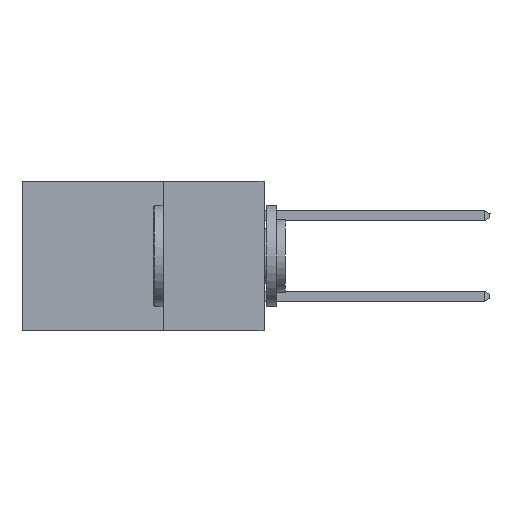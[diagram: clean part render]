
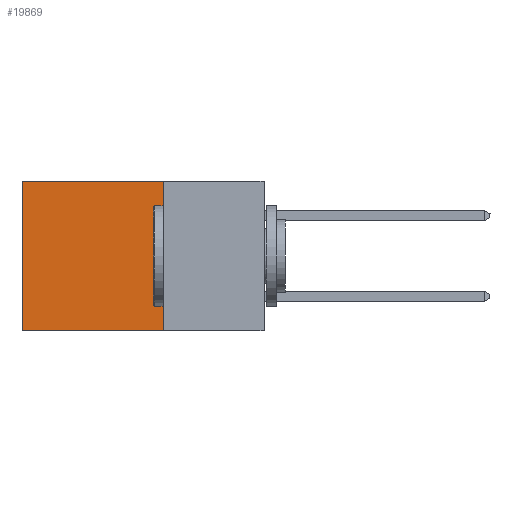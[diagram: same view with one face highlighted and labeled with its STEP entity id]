
A CAD part, left-side view. The second image highlights one B-rep face of the part: STEP entity #19869.
In plain terms, the highlighted planar face has unit normal (-1, 0, 0).
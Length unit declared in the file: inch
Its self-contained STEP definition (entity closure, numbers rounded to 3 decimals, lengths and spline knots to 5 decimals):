
#702 = CARTESIAN_POINT ( 'NONE',  ( 0.298, 0.25, 0. ) ) ;
#1252 = CARTESIAN_POINT ( 'NONE',  ( 0.298, 0.25, 0. ) ) ;
#1754 = ORIENTED_EDGE ( 'NONE', *, *, #15836, .T. ) ;
#6641 = EDGE_LOOP ( 'NONE', ( #19801, #10557, #20972, #1754 ) ) ;
#7192 = DIRECTION ( 'NONE',  ( 0., 0., -1. ) ) ;
#8201 = LINE ( 'NONE', #23012, #13774 ) ;
#8579 = LINE ( 'NONE', #20771, #9980 ) ;
#9673 = LINE ( 'NONE', #11593, #13516 ) ;
#9980 = VECTOR ( 'NONE', #27638, 39.37008 ) ;
#10557 = ORIENTED_EDGE ( 'NONE', *, *, #11553, .F. ) ;
#10643 = FACE_OUTER_BOUND ( 'NONE', #6641, .T. ) ;
#11553 = EDGE_CURVE ( 'NONE', #19592, #14748, #8579, .T. ) ;
#11593 = CARTESIAN_POINT ( 'NONE',  ( 0.298, 0.25, 0. ) ) ;
#12552 = CARTESIAN_POINT ( 'NONE',  ( 0.298, 0.25, -0.37 ) ) ;
#13516 = VECTOR ( 'NONE', #7192, 39.37008 ) ;
#13774 = VECTOR ( 'NONE', #25416, 39.37008 ) ;
#14577 = DIRECTION ( 'NONE',  ( 1., 0., 0. ) ) ;
#14748 = VERTEX_POINT ( 'NONE', #20721 ) ;
#14956 = LINE ( 'NONE', #702, #27445 ) ;
#15033 = DIRECTION ( 'NONE',  ( 0., 1., 0. ) ) ;
#15515 = VERTEX_POINT ( 'NONE', #25421 ) ;
#15836 = EDGE_CURVE ( 'NONE', #15515, #22564, #14956, .T. ) ;
#19592 = VERTEX_POINT ( 'NONE', #12552 ) ;
#19801 = ORIENTED_EDGE ( 'NONE', *, *, #25153, .T. ) ;
#19869 = ADVANCED_FACE ( 'NONE', ( #10643 ), #23320, .F. ) ;
#20632 = AXIS2_PLACEMENT_3D ( 'NONE', #1252, #14577, #21442 ) ;
#20721 = CARTESIAN_POINT ( 'NONE',  ( 0.298, 0.6, -0.37 ) ) ;
#20771 = CARTESIAN_POINT ( 'NONE',  ( 0.298, 0.25, -0.37 ) ) ;
#20972 = ORIENTED_EDGE ( 'NONE', *, *, #23958, .F. ) ;
#21442 = DIRECTION ( 'NONE',  ( 0., 0., -1. ) ) ;
#22564 = VERTEX_POINT ( 'NONE', #24837 ) ;
#23012 = CARTESIAN_POINT ( 'NONE',  ( 0.298, 0.6, 0. ) ) ;
#23320 = PLANE ( 'NONE',  #20632 ) ;
#23958 = EDGE_CURVE ( 'NONE', #15515, #19592, #9673, .T. ) ;
#24837 = CARTESIAN_POINT ( 'NONE',  ( 0.298, 0.6, 0. ) ) ;
#25153 = EDGE_CURVE ( 'NONE', #22564, #14748, #8201, .T. ) ;
#25416 = DIRECTION ( 'NONE',  ( 0., 0., -1. ) ) ;
#25421 = CARTESIAN_POINT ( 'NONE',  ( 0.298, 0.25, 0. ) ) ;
#27445 = VECTOR ( 'NONE', #15033, 39.37008 ) ;
#27638 = DIRECTION ( 'NONE',  ( 0., 1., 0. ) ) ;
